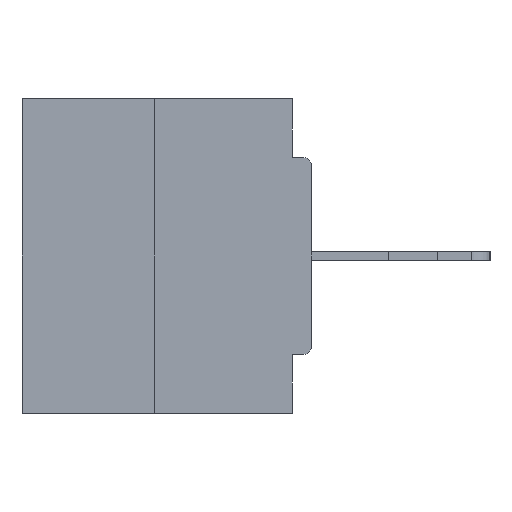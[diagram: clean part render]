
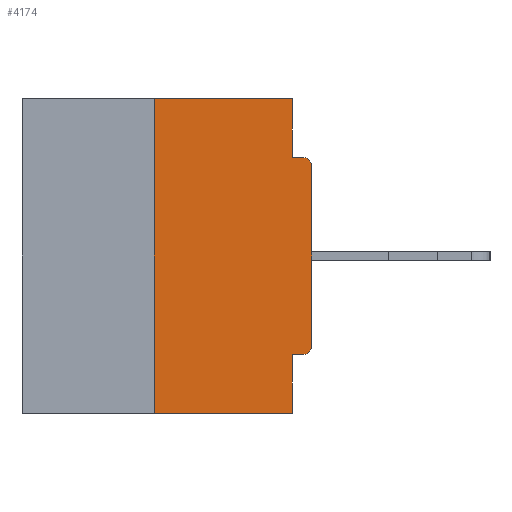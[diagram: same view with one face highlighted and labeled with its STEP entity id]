
A CAD part, left-side view. The second image highlights one B-rep face of the part: STEP entity #4174.
In plain terms, the highlighted planar face has unit normal (-1, 0, 0).
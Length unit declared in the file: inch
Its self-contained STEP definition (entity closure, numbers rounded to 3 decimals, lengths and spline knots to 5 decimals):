
#379 = VECTOR ( 'NONE', #21420, 39.37008 ) ;
#595 = EDGE_CURVE ( 'NONE', #15964, #11702, #17959, .T. ) ;
#1018 = CARTESIAN_POINT ( 'NONE',  ( 0., 0.015, -0.1085 ) ) ;
#1657 = VERTEX_POINT ( 'NONE', #34206 ) ;
#2023 = DIRECTION ( 'NONE',  ( 0., 0., -1. ) ) ;
#3076 = EDGE_CURVE ( 'NONE', #33101, #29836, #23779, .T. ) ;
#3167 = DIRECTION ( 'NONE',  ( 1., 0., 0. ) ) ;
#3636 = DIRECTION ( 'NONE',  ( 0., 0., -1. ) ) ;
#4113 = DIRECTION ( 'NONE',  ( -1., 0., 0. ) ) ;
#4174 = ADVANCED_FACE ( 'NONE', ( #6635 ), #21099, .F. ) ;
#4183 = VECTOR ( 'NONE', #9173, 39.37008 ) ;
#4239 = VERTEX_POINT ( 'NONE', #24207 ) ;
#5298 = EDGE_LOOP ( 'NONE', ( #7519, #18178, #5758, #36473, #24072, #10436, #25171, #22113, #10581, #23565 ) ) ;
#5374 = CARTESIAN_POINT ( 'NONE',  ( 0., 0., -0.1085 ) ) ;
#5758 = ORIENTED_EDGE ( 'NONE', *, *, #595, .T. ) ;
#6533 = EDGE_CURVE ( 'NONE', #26720, #21295, #32526, .T. ) ;
#6567 = CARTESIAN_POINT ( 'NONE',  ( 0., 0.46, -0.5 ) ) ;
#6635 = FACE_OUTER_BOUND ( 'NONE', #5298, .T. ) ;
#7519 = ORIENTED_EDGE ( 'NONE', *, *, #10732, .F. ) ;
#9173 = DIRECTION ( 'NONE',  ( 0., 0., 1. ) ) ;
#9536 = EDGE_CURVE ( 'NONE', #21295, #34293, #24111, .T. ) ;
#10436 = ORIENTED_EDGE ( 'NONE', *, *, #16045, .T. ) ;
#10456 = CARTESIAN_POINT ( 'NONE',  ( 0., 0.031, -0.0935 ) ) ;
#10520 = LINE ( 'NONE', #28470, #32972 ) ;
#10581 = ORIENTED_EDGE ( 'NONE', *, *, #11171, .F. ) ;
#10732 = EDGE_CURVE ( 'NONE', #1657, #33101, #31596, .T. ) ;
#10851 = LINE ( 'NONE', #13577, #26689 ) ;
#11171 = EDGE_CURVE ( 'NONE', #29836, #34293, #27289, .T. ) ;
#11399 = CARTESIAN_POINT ( 'NONE',  ( 0., 0.015, -0.0935 ) ) ;
#11702 = VERTEX_POINT ( 'NONE', #33678 ) ;
#12247 = DIRECTION ( 'NONE',  ( 0., 0., -1. ) ) ;
#12249 = CARTESIAN_POINT ( 'NONE',  ( 0., 0., -0.0935 ) ) ;
#13577 = CARTESIAN_POINT ( 'NONE',  ( 0., 0.25, 0. ) ) ;
#14442 = VECTOR ( 'NONE', #30511, 39.37008 ) ;
#14795 = EDGE_CURVE ( 'NONE', #4239, #11702, #10520, .T. ) ;
#15964 = VERTEX_POINT ( 'NONE', #35885 ) ;
#16045 = EDGE_CURVE ( 'NONE', #26454, #26720, #23091, .T. ) ;
#17959 = LINE ( 'NONE', #6567, #379 ) ;
#18101 = LINE ( 'NONE', #36422, #34196 ) ;
#18178 = ORIENTED_EDGE ( 'NONE', *, *, #27009, .F. ) ;
#21099 = PLANE ( 'NONE',  #37308 ) ;
#21295 = VERTEX_POINT ( 'NONE', #5374 ) ;
#21420 = DIRECTION ( 'NONE',  ( 0., -1., 0. ) ) ;
#22113 = ORIENTED_EDGE ( 'NONE', *, *, #9536, .T. ) ;
#23091 = CIRCLE ( 'NONE', #28033, 0.015 ) ;
#23450 = CARTESIAN_POINT ( 'NONE',  ( 0., 0., 0. ) ) ;
#23529 = CARTESIAN_POINT ( 'NONE',  ( 0., 0.015, -0.3915 ) ) ;
#23565 = ORIENTED_EDGE ( 'NONE', *, *, #3076, .F. ) ;
#23779 = LINE ( 'NONE', #35558, #14442 ) ;
#24072 = ORIENTED_EDGE ( 'NONE', *, *, #29505, .F. ) ;
#24111 = CIRCLE ( 'NONE', #33362, 0.015 ) ;
#24198 = DIRECTION ( 'NONE',  ( 0., 0., -1. ) ) ;
#24207 = CARTESIAN_POINT ( 'NONE',  ( 0., 0.031, -0.4065 ) ) ;
#24288 = DIRECTION ( 'NONE',  ( -1., 0., 0. ) ) ;
#25171 = ORIENTED_EDGE ( 'NONE', *, *, #6533, .T. ) ;
#25548 = DIRECTION ( 'NONE',  ( 0., 0., 1. ) ) ;
#26454 = VERTEX_POINT ( 'NONE', #27336 ) ;
#26689 = VECTOR ( 'NONE', #25548, 39.37008 ) ;
#26720 = VERTEX_POINT ( 'NONE', #32712 ) ;
#26793 = CARTESIAN_POINT ( 'NONE',  ( 0., 0.031, 0. ) ) ;
#27009 = EDGE_CURVE ( 'NONE', #15964, #1657, #10851, .T. ) ;
#27289 = LINE ( 'NONE', #12249, #30913 ) ;
#27336 = CARTESIAN_POINT ( 'NONE',  ( 0., 0.015, -0.4065 ) ) ;
#28033 = AXIS2_PLACEMENT_3D ( 'NONE', #23529, #24288, #3636 ) ;
#28470 = CARTESIAN_POINT ( 'NONE',  ( 0., 0.031, -0.5 ) ) ;
#28701 = CARTESIAN_POINT ( 'NONE',  ( 0., 0.46, 0. ) ) ;
#29505 = EDGE_CURVE ( 'NONE', #26454, #4239, #18101, .T. ) ;
#29612 = CARTESIAN_POINT ( 'NONE',  ( 0., 0.46, 0. ) ) ;
#29637 = VECTOR ( 'NONE', #37572, 39.37008 ) ;
#29836 = VERTEX_POINT ( 'NONE', #10456 ) ;
#30511 = DIRECTION ( 'NONE',  ( 0., 0., -1. ) ) ;
#30913 = VECTOR ( 'NONE', #32519, 39.37008 ) ;
#31596 = LINE ( 'NONE', #28701, #29637 ) ;
#32519 = DIRECTION ( 'NONE',  ( 0., -1., 0. ) ) ;
#32526 = LINE ( 'NONE', #23450, #4183 ) ;
#32712 = CARTESIAN_POINT ( 'NONE',  ( 0., 0., -0.3915 ) ) ;
#32775 = DIRECTION ( 'NONE',  ( 0., 1., 0. ) ) ;
#32972 = VECTOR ( 'NONE', #2023, 39.37008 ) ;
#33101 = VERTEX_POINT ( 'NONE', #26793 ) ;
#33362 = AXIS2_PLACEMENT_3D ( 'NONE', #1018, #4113, #24198 ) ;
#33678 = CARTESIAN_POINT ( 'NONE',  ( 0., 0.031, -0.5 ) ) ;
#34196 = VECTOR ( 'NONE', #32775, 39.37008 ) ;
#34206 = CARTESIAN_POINT ( 'NONE',  ( 0., 0.25, 0. ) ) ;
#34293 = VERTEX_POINT ( 'NONE', #11399 ) ;
#35558 = CARTESIAN_POINT ( 'NONE',  ( 0., 0.031, 0. ) ) ;
#35885 = CARTESIAN_POINT ( 'NONE',  ( 0., 0.25, -0.5 ) ) ;
#36422 = CARTESIAN_POINT ( 'NONE',  ( 0., 0., -0.4065 ) ) ;
#36473 = ORIENTED_EDGE ( 'NONE', *, *, #14795, .F. ) ;
#37308 = AXIS2_PLACEMENT_3D ( 'NONE', #29612, #3167, #12247 ) ;
#37572 = DIRECTION ( 'NONE',  ( 0., -1., 0. ) ) ;
